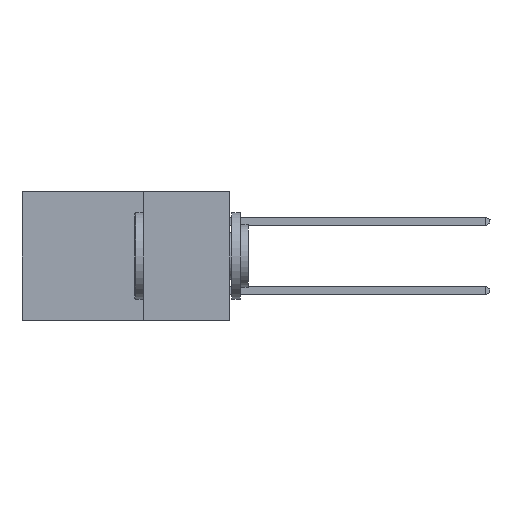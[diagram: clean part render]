
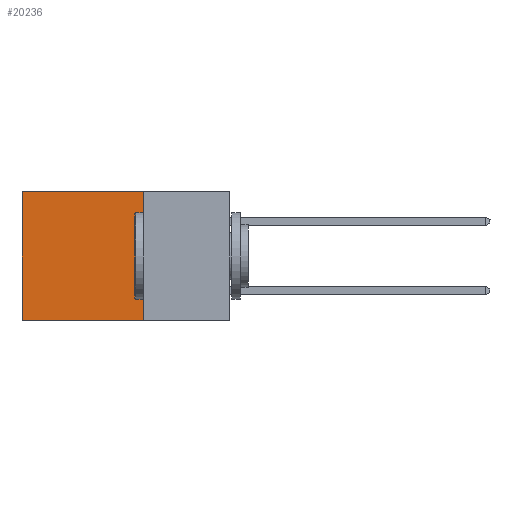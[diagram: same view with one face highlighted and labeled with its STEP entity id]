
A CAD part, left-side view. The second image highlights one B-rep face of the part: STEP entity #20236.
In plain terms, the highlighted planar face has unit normal (-1, 0, 0).
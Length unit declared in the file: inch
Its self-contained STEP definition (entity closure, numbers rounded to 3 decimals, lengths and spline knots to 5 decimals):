
#1132 = VERTEX_POINT ( 'NONE', #11471 ) ;
#1243 = CARTESIAN_POINT ( 'NONE',  ( 0.2615, 0.6, 0. ) ) ;
#2115 = VECTOR ( 'NONE', #23837, 39.37008 ) ;
#3242 = VERTEX_POINT ( 'NONE', #20631 ) ;
#4403 = DIRECTION ( 'NONE',  ( 0., 0., -1. ) ) ;
#4862 = EDGE_LOOP ( 'NONE', ( #6985, #21621, #7345, #7525 ) ) ;
#5155 = CARTESIAN_POINT ( 'NONE',  ( 0.2615, 0.25, -0.37 ) ) ;
#5393 = LINE ( 'NONE', #5155, #2115 ) ;
#5784 = EDGE_CURVE ( 'NONE', #23402, #15009, #12015, .T. ) ;
#6116 = FACE_OUTER_BOUND ( 'NONE', #4862, .T. ) ;
#6985 = ORIENTED_EDGE ( 'NONE', *, *, #15855, .T. ) ;
#7181 = EDGE_CURVE ( 'NONE', #23402, #3242, #5393, .T. ) ;
#7345 = ORIENTED_EDGE ( 'NONE', *, *, #7181, .F. ) ;
#7525 = ORIENTED_EDGE ( 'NONE', *, *, #5784, .T. ) ;
#8479 = DIRECTION ( 'NONE',  ( 0., 1., 0. ) ) ;
#9781 = CARTESIAN_POINT ( 'NONE',  ( 0.2615, 0.25, -0.37 ) ) ;
#10492 = VECTOR ( 'NONE', #11633, 39.37008 ) ;
#11471 = CARTESIAN_POINT ( 'NONE',  ( 0.2615, 0.6, -0.37 ) ) ;
#11633 = DIRECTION ( 'NONE',  ( 0., 1., 0. ) ) ;
#11873 = CARTESIAN_POINT ( 'NONE',  ( 0.2615, 0.25, -0.37 ) ) ;
#12015 = LINE ( 'NONE', #19442, #23195 ) ;
#12021 = DIRECTION ( 'NONE',  ( 0., 0., -1. ) ) ;
#12754 = EDGE_CURVE ( 'NONE', #3242, #1132, #15655, .T. ) ;
#13240 = VECTOR ( 'NONE', #12021, 39.37008 ) ;
#13561 = DIRECTION ( 'NONE',  ( 1., 0., 0. ) ) ;
#13853 = LINE ( 'NONE', #21315, #13240 ) ;
#14464 = AXIS2_PLACEMENT_3D ( 'NONE', #9781, #13561, #4403 ) ;
#15009 = VERTEX_POINT ( 'NONE', #1243 ) ;
#15030 = PLANE ( 'NONE',  #14464 ) ;
#15655 = LINE ( 'NONE', #11873, #10492 ) ;
#15855 = EDGE_CURVE ( 'NONE', #15009, #1132, #13853, .T. ) ;
#16633 = CARTESIAN_POINT ( 'NONE',  ( 0.2615, 0.25, 0. ) ) ;
#19442 = CARTESIAN_POINT ( 'NONE',  ( 0.2615, 0.25, 0. ) ) ;
#20236 = ADVANCED_FACE ( 'NONE', ( #6116 ), #15030, .F. ) ;
#20631 = CARTESIAN_POINT ( 'NONE',  ( 0.2615, 0.25, -0.37 ) ) ;
#21315 = CARTESIAN_POINT ( 'NONE',  ( 0.2615, 0.6, -0.37 ) ) ;
#21621 = ORIENTED_EDGE ( 'NONE', *, *, #12754, .F. ) ;
#23195 = VECTOR ( 'NONE', #8479, 39.37008 ) ;
#23402 = VERTEX_POINT ( 'NONE', #16633 ) ;
#23837 = DIRECTION ( 'NONE',  ( 0., 0., -1. ) ) ;
